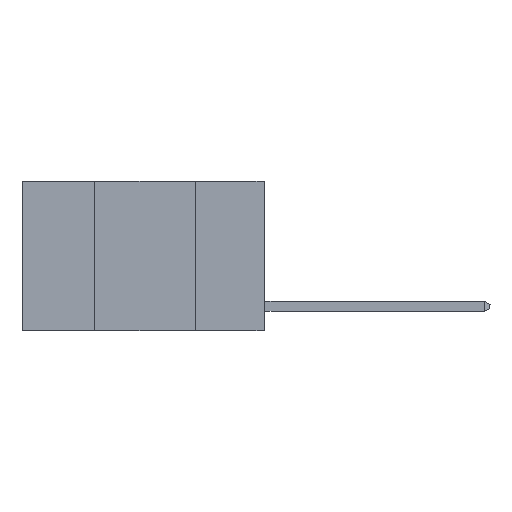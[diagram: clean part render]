
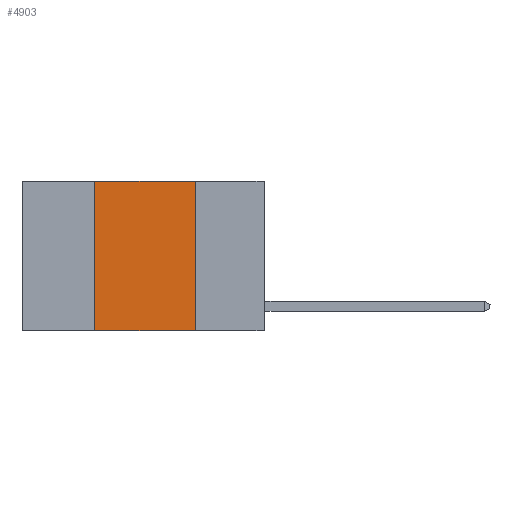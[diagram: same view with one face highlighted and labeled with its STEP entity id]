
A CAD part, left-side view. The second image highlights one B-rep face of the part: STEP entity #4903.
In plain terms, the highlighted planar face has unit normal (-1, 0, 0).
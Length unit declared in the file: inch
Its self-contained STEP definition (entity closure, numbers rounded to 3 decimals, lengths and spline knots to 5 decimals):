
#286 = CARTESIAN_POINT ( 'NONE',  ( 0., 0.6, 0. ) ) ;
#326 = CARTESIAN_POINT ( 'NONE',  ( 0., 0.17, -0.37 ) ) ;
#1812 = ORIENTED_EDGE ( 'NONE', *, *, #5290, .F. ) ;
#1920 = LINE ( 'NONE', #9442, #10025 ) ;
#1922 = EDGE_LOOP ( 'NONE', ( #3768, #1812, #10399, #2065 ) ) ;
#2065 = ORIENTED_EDGE ( 'NONE', *, *, #10825, .T. ) ;
#2366 = DIRECTION ( 'NONE',  ( 0., 0., 1. ) ) ;
#2641 = LINE ( 'NONE', #6149, #7440 ) ;
#2684 = DIRECTION ( 'NONE',  ( 0., 0., -1. ) ) ;
#2732 = CARTESIAN_POINT ( 'NONE',  ( 0., 0.42, 0. ) ) ;
#3184 = VERTEX_POINT ( 'NONE', #326 ) ;
#3768 = ORIENTED_EDGE ( 'NONE', *, *, #9279, .F. ) ;
#4232 = CARTESIAN_POINT ( 'NONE',  ( 0., 0.6, -0.37 ) ) ;
#4273 = DIRECTION ( 'NONE',  ( 0., -1., 0. ) ) ;
#4615 = VECTOR ( 'NONE', #7181, 39.37008 ) ;
#4678 = VECTOR ( 'NONE', #4273, 39.37008 ) ;
#4903 = ADVANCED_FACE ( 'NONE', ( #6098 ), #11624, .F. ) ;
#5290 = EDGE_CURVE ( 'NONE', #8215, #7915, #9901, .T. ) ;
#5326 = CARTESIAN_POINT ( 'NONE',  ( 0., 0.6, 0. ) ) ;
#6098 = FACE_OUTER_BOUND ( 'NONE', #1922, .T. ) ;
#6149 = CARTESIAN_POINT ( 'NONE',  ( 0., 0.17, 0. ) ) ;
#6486 = CARTESIAN_POINT ( 'NONE',  ( 0., 0.42, -0.37 ) ) ;
#7181 = DIRECTION ( 'NONE',  ( 0., -1., 0. ) ) ;
#7440 = VECTOR ( 'NONE', #12968, 39.37008 ) ;
#7915 = VERTEX_POINT ( 'NONE', #11102 ) ;
#8215 = VERTEX_POINT ( 'NONE', #2732 ) ;
#8746 = DIRECTION ( 'NONE',  ( 1., 0., 0. ) ) ;
#8895 = EDGE_CURVE ( 'NONE', #13132, #8215, #1920, .T. ) ;
#9279 = EDGE_CURVE ( 'NONE', #7915, #3184, #2641, .T. ) ;
#9442 = CARTESIAN_POINT ( 'NONE',  ( 0., 0.42, 0. ) ) ;
#9566 = AXIS2_PLACEMENT_3D ( 'NONE', #286, #8746, #2684 ) ;
#9843 = LINE ( 'NONE', #4232, #4615 ) ;
#9901 = LINE ( 'NONE', #5326, #4678 ) ;
#10025 = VECTOR ( 'NONE', #2366, 39.37008 ) ;
#10399 = ORIENTED_EDGE ( 'NONE', *, *, #8895, .F. ) ;
#10825 = EDGE_CURVE ( 'NONE', #13132, #3184, #9843, .T. ) ;
#11102 = CARTESIAN_POINT ( 'NONE',  ( 0., 0.17, 0. ) ) ;
#11624 = PLANE ( 'NONE',  #9566 ) ;
#12968 = DIRECTION ( 'NONE',  ( 0., 0., -1. ) ) ;
#13132 = VERTEX_POINT ( 'NONE', #6486 ) ;
